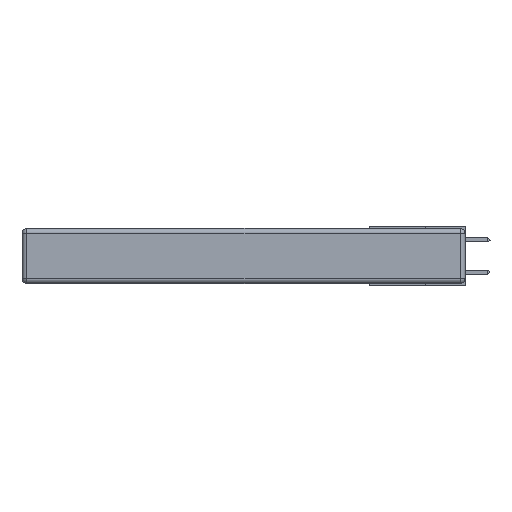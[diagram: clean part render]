
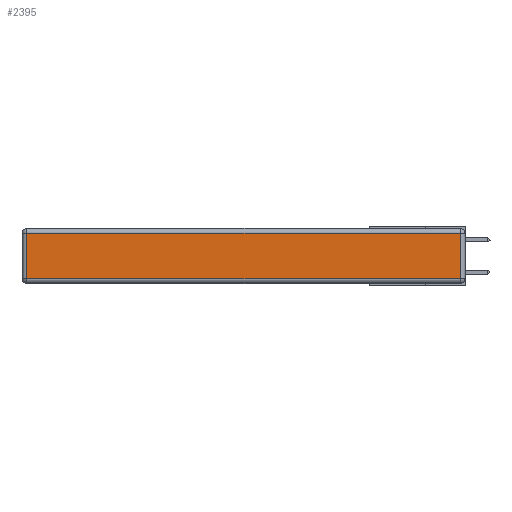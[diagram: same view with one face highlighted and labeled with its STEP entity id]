
A CAD part, left-side view. The second image highlights one B-rep face of the part: STEP entity #2395.
In plain terms, the highlighted planar face has unit normal (-1, 0, 0).
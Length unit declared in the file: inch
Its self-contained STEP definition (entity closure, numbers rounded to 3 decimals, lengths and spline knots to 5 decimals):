
#288 = LINE ( 'NONE', #15770, #16562 ) ;
#1286 = CARTESIAN_POINT ( 'NONE',  ( 0., 2.72, -0.03 ) ) ;
#1748 = LINE ( 'NONE', #8486, #16587 ) ;
#2395 = ADVANCED_FACE ( 'NONE', ( #7286 ), #4025, .T. ) ;
#2811 = EDGE_CURVE ( 'NONE', #4834, #3151, #11478, .T. ) ;
#2931 = DIRECTION ( 'NONE',  ( 0., 0., 1. ) ) ;
#2971 = CARTESIAN_POINT ( 'NONE',  ( 0., 2.72, -0.313 ) ) ;
#3151 = VERTEX_POINT ( 'NONE', #1286 ) ;
#4025 = PLANE ( 'NONE',  #15015 ) ;
#4212 = VERTEX_POINT ( 'NONE', #2971 ) ;
#4668 = VECTOR ( 'NONE', #15205, 39.37008 ) ;
#4834 = VERTEX_POINT ( 'NONE', #5620 ) ;
#5122 = CARTESIAN_POINT ( 'NONE',  ( 0., 0., -0.343 ) ) ;
#5308 = LINE ( 'NONE', #10056, #12303 ) ;
#5620 = CARTESIAN_POINT ( 'NONE',  ( 0., 0.03, -0.03 ) ) ;
#6565 = ORIENTED_EDGE ( 'NONE', *, *, #2811, .T. ) ;
#7286 = FACE_OUTER_BOUND ( 'NONE', #12543, .T. ) ;
#8486 = CARTESIAN_POINT ( 'NONE',  ( 0., 0., -0.313 ) ) ;
#10056 = CARTESIAN_POINT ( 'NONE',  ( 0., 2.72, -0.343 ) ) ;
#10225 = CARTESIAN_POINT ( 'NONE',  ( 0., 2.75, -0.03 ) ) ;
#10699 = DIRECTION ( 'NONE',  ( 0., 0., 1. ) ) ;
#11330 = DIRECTION ( 'NONE',  ( 0., 0., -1. ) ) ;
#11478 = LINE ( 'NONE', #10225, #4668 ) ;
#12303 = VECTOR ( 'NONE', #11330, 39.37008 ) ;
#12315 = EDGE_CURVE ( 'NONE', #4212, #14798, #1748, .T. ) ;
#12543 = EDGE_LOOP ( 'NONE', ( #13003, #15181, #6565, #13704 ) ) ;
#12579 = EDGE_CURVE ( 'NONE', #14798, #4834, #288, .T. ) ;
#12971 = DIRECTION ( 'NONE',  ( -1., 0., 0. ) ) ;
#13003 = ORIENTED_EDGE ( 'NONE', *, *, #12315, .T. ) ;
#13704 = ORIENTED_EDGE ( 'NONE', *, *, #14605, .T. ) ;
#14605 = EDGE_CURVE ( 'NONE', #3151, #4212, #5308, .T. ) ;
#14695 = CARTESIAN_POINT ( 'NONE',  ( 0., 0.03, -0.313 ) ) ;
#14798 = VERTEX_POINT ( 'NONE', #14695 ) ;
#15015 = AXIS2_PLACEMENT_3D ( 'NONE', #5122, #12971, #10699 ) ;
#15181 = ORIENTED_EDGE ( 'NONE', *, *, #12579, .T. ) ;
#15205 = DIRECTION ( 'NONE',  ( 0., 1., 0. ) ) ;
#15770 = CARTESIAN_POINT ( 'NONE',  ( 0., 0.03, -0.343 ) ) ;
#16190 = DIRECTION ( 'NONE',  ( 0., -1., 0. ) ) ;
#16562 = VECTOR ( 'NONE', #2931, 39.37008 ) ;
#16587 = VECTOR ( 'NONE', #16190, 39.37008 ) ;
